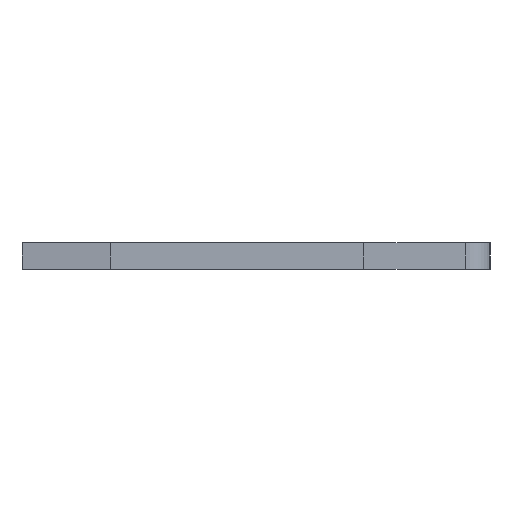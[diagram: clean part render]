
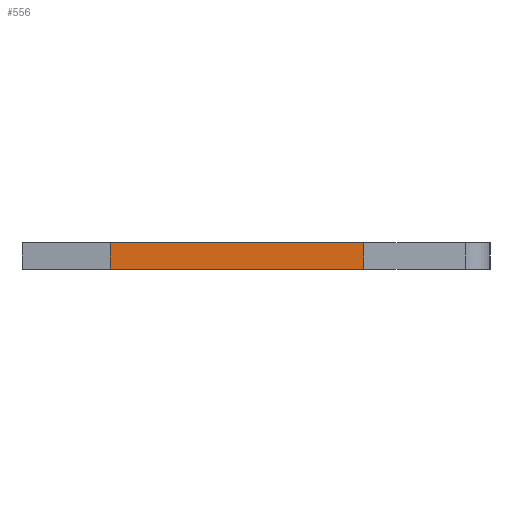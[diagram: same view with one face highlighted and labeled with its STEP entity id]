
A CAD part, left-side view. The second image highlights one B-rep face of the part: STEP entity #556.
In plain terms, the highlighted face is planar.
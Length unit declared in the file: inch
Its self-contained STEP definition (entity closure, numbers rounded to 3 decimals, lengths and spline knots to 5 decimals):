
#13 = VERTEX_POINT ( 'NONE', #1569 ) ;
#16 = FACE_OUTER_BOUND ( 'NONE', #600, .T. ) ;
#170 = CARTESIAN_POINT ( 'NONE',  ( 0.013, -0.099, -0.0575 ) ) ;
#177 = DIRECTION ( 'NONE',  ( -1., 0., 0. ) ) ;
#189 = VECTOR ( 'NONE', #427, 39.37008 ) ;
#235 = CARTESIAN_POINT ( 'NONE',  ( -0.013, -0.099, -0.0575 ) ) ;
#248 = VECTOR ( 'NONE', #932, 39.37008 ) ;
#278 = CARTESIAN_POINT ( 'NONE',  ( 0.013, 0.146, -0.0575 ) ) ;
#315 = VECTOR ( 'NONE', #177, 39.37008 ) ;
#360 = ORIENTED_EDGE ( 'NONE', *, *, #1091, .F. ) ;
#427 = DIRECTION ( 'NONE',  ( 0., 1., 0. ) ) ;
#551 = ORIENTED_EDGE ( 'NONE', *, *, #1242, .T. ) ;
#556 = ADVANCED_FACE ( 'NONE', ( #16 ), #1530, .F. ) ;
#599 = EDGE_CURVE ( 'NONE', #1654, #13, #1384, .T. ) ;
#600 = EDGE_LOOP ( 'NONE', ( #1155, #1234, #360, #551 ) ) ;
#604 = LINE ( 'NONE', #1329, #248 ) ;
#860 = CARTESIAN_POINT ( 'NONE',  ( 0.013, 0.146, -0.0575 ) ) ;
#867 = EDGE_CURVE ( 'NONE', #1181, #13, #604, .T. ) ;
#932 = DIRECTION ( 'NONE',  ( -1., 0., 0. ) ) ;
#985 = CARTESIAN_POINT ( 'NONE',  ( 0.013, -0.099, -0.0575 ) ) ;
#996 = DIRECTION ( 'NONE',  ( 0., 0., 1. ) ) ;
#1025 = CARTESIAN_POINT ( 'NONE',  ( -0.013, 0.146, -0.0575 ) ) ;
#1091 = EDGE_CURVE ( 'NONE', #1338, #1181, #1553, .T. ) ;
#1155 = ORIENTED_EDGE ( 'NONE', *, *, #599, .T. ) ;
#1181 = VERTEX_POINT ( 'NONE', #1253 ) ;
#1234 = ORIENTED_EDGE ( 'NONE', *, *, #867, .F. ) ;
#1242 = EDGE_CURVE ( 'NONE', #1338, #1654, #1248, .T. ) ;
#1248 = LINE ( 'NONE', #985, #315 ) ;
#1253 = CARTESIAN_POINT ( 'NONE',  ( 0.013, 0.146, -0.0575 ) ) ;
#1314 = VECTOR ( 'NONE', #1540, 39.37008 ) ;
#1329 = CARTESIAN_POINT ( 'NONE',  ( 0.013, 0.146, -0.0575 ) ) ;
#1338 = VERTEX_POINT ( 'NONE', #170 ) ;
#1362 = AXIS2_PLACEMENT_3D ( 'NONE', #860, #996, #1368 ) ;
#1368 = DIRECTION ( 'NONE',  ( 1., 0., 0. ) ) ;
#1384 = LINE ( 'NONE', #1025, #1314 ) ;
#1530 = PLANE ( 'NONE',  #1362 ) ;
#1540 = DIRECTION ( 'NONE',  ( 0., 1., 0. ) ) ;
#1553 = LINE ( 'NONE', #278, #189 ) ;
#1569 = CARTESIAN_POINT ( 'NONE',  ( -0.013, 0.146, -0.0575 ) ) ;
#1654 = VERTEX_POINT ( 'NONE', #235 ) ;
